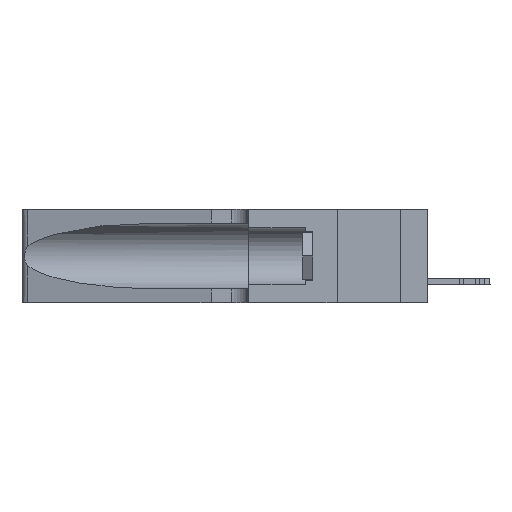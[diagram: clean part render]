
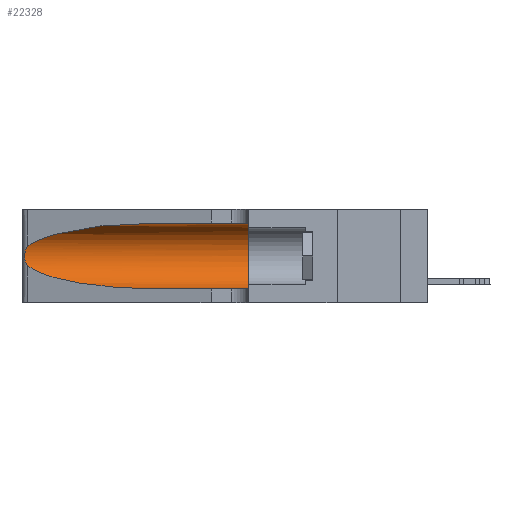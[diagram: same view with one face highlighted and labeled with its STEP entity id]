
A CAD part, left-side view. The second image highlights one B-rep face of the part: STEP entity #22328.
In plain terms, the highlighted cylindrical face has radius 3.308 mm (diameter 6.617 mm), a partial arc.
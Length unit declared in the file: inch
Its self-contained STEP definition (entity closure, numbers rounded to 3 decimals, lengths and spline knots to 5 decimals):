
#170 = CARTESIAN_POINT ( 'NONE',  ( 0.1305, 0.72297, 0.05475 ) ) ;
#657 = LINE ( 'NONE', #12753, #15418 ) ;
#1039 = CARTESIAN_POINT ( 'NONE',  ( 0.25487, 1.22718, 0.14631 ) ) ;
#1670 = VERTEX_POINT ( 'NONE', #14358 ) ;
#2131 = AXIS2_PLACEMENT_3D ( 'NONE', #8786, #8942, #35774 ) ;
#4303 = EDGE_CURVE ( 'NONE', #12746, #25970, #12121, .T. ) ;
#4893 = CARTESIAN_POINT ( 'NONE',  ( 0.26018, 1.23835, 0.19895 ) ) ;
#6240 = FACE_OUTER_BOUND ( 'NONE', #11976, .T. ) ;
#8786 = CARTESIAN_POINT ( 'NONE',  ( 0.1305, 0.35, 0.185 ) ) ;
#8942 = DIRECTION ( 'NONE',  ( 0., 1., 0. ) ) ;
#9228 = DIRECTION ( 'NONE',  ( 0., -1., 0. ) ) ;
#10283 = ORIENTED_EDGE ( 'NONE', *, *, #4303, .F. ) ;
#11208 = DIRECTION ( 'NONE',  ( 0., -1., 0. ) ) ;
#11501 = CARTESIAN_POINT ( 'NONE',  ( 0.26017, 1.23833, 0.17102 ) ) ;
#11976 = EDGE_LOOP ( 'NONE', ( #29747, #21127, #13258, #29971, #10283, #15335 ) ) ;
#12121 = CIRCLE ( 'NONE', #2131, 0.13025 ) ;
#12572 = VERTEX_POINT ( 'NONE', #23150 ) ;
#12648 = VERTEX_POINT ( 'NONE', #15117 ) ;
#12746 = VERTEX_POINT ( 'NONE', #41838 ) ;
#12753 = CARTESIAN_POINT ( 'NONE',  ( 0.1305, 1.61858, 0.05475 ) ) ;
#13258 = ORIENTED_EDGE ( 'NONE', *, *, #41507, .T. ) ;
#13763 = CARTESIAN_POINT ( 'NONE',  ( 0.1305, 0.72297, 0.31525 ) ) ;
#14358 = CARTESIAN_POINT ( 'NONE',  ( 0.25487, 1.22718, 0.14631 ) ) ;
#14885 = CARTESIAN_POINT ( 'NONE',  ( 0.25789, 1.23486, 0.15765 ) ) ;
#15117 = CARTESIAN_POINT ( 'NONE',  ( 0.25487, 1.22718, 0.22369 ) ) ;
#15335 = ORIENTED_EDGE ( 'NONE', *, *, #25459, .F. ) ;
#15418 = VECTOR ( 'NONE', #9228, 39.37008 ) ;
#16568 = LINE ( 'NONE', #31150, #32900 ) ;
#16634 = CARTESIAN_POINT ( 'NONE',  ( 0.18966, 0.96281, 0.31525 ) ) ;
#17762 = B_SPLINE_CURVE_WITH_KNOTS ( 'NONE', 3,
 ( #21868, #42118, #39004, #28950, #18759, #4893, #42271, #35710, #11501, #32197, #14885, #18617, #18314, #42435 ),
 .UNSPECIFIED., .F., .F.,
 ( 4, 2, 2, 2, 2, 2, 4 ),
 ( 0., 0.00027, 0.00053, 0.00107, 0.0016, 0.00187, 0.00214 ),
 .UNSPECIFIED. ) ;
#17767 = CYLINDRICAL_SURFACE ( 'NONE', #22384, 0.13025 ) ;
#18314 = CARTESIAN_POINT ( 'NONE',  ( 0.25555, 1.22993, 0.14849 ) ) ;
#18617 = CARTESIAN_POINT ( 'NONE',  ( 0.25639, 1.23186, 0.15144 ) ) ;
#18759 = CARTESIAN_POINT ( 'NONE',  ( 0.25854, 1.2359, 0.20912 ) ) ;
#19297 = CARTESIAN_POINT ( 'NONE',  ( 0.1305, 0.35, 0.05475 ) ) ;
#19692 = EDGE_CURVE ( 'NONE', #12572, #25970, #657, .T. ) ;
#20511 =( BOUNDED_CURVE ( )  B_SPLINE_CURVE ( 3, ( #1039, #24643, #34062, #170 ),
 .UNSPECIFIED., .F., .F. ) 
 B_SPLINE_CURVE_WITH_KNOTS ( ( 4, 4 ),
 ( 3.44316, 4.71239 ),
 .UNSPECIFIED. ) 
 CURVE ( )  GEOMETRIC_REPRESENTATION_ITEM ( )  RATIONAL_B_SPLINE_CURVE ( ( 1., 0.87, 0.87, 1. ) ) 
 REPRESENTATION_ITEM ( '' )  );
#21127 = ORIENTED_EDGE ( 'NONE', *, *, #36925, .T. ) ;
#21868 = CARTESIAN_POINT ( 'NONE',  ( 0.25487, 1.22718, 0.22369 ) ) ;
#22328 = ADVANCED_FACE ( 'NONE', ( #6240 ), #17767, .F. ) ;
#22384 = AXIS2_PLACEMENT_3D ( 'NONE', #37200, #41311, #41622 ) ;
#23150 = CARTESIAN_POINT ( 'NONE',  ( 0.1305, 0.72297, 0.05475 ) ) ;
#24643 = CARTESIAN_POINT ( 'NONE',  ( 0.2373, 1.15595, 0.08982 ) ) ;
#25459 = EDGE_CURVE ( 'NONE', #35437, #12746, #16568, .T. ) ;
#25970 = VERTEX_POINT ( 'NONE', #19297 ) ;
#28950 = CARTESIAN_POINT ( 'NONE',  ( 0.25787, 1.23484, 0.2124 ) ) ;
#29747 = ORIENTED_EDGE ( 'NONE', *, *, #37777, .T. ) ;
#29971 = ORIENTED_EDGE ( 'NONE', *, *, #19692, .T. ) ;
#30467 = CARTESIAN_POINT ( 'NONE',  ( 0.25487, 1.22718, 0.22369 ) ) ;
#31150 = CARTESIAN_POINT ( 'NONE',  ( 0.1305, 1.61858, 0.31525 ) ) ;
#32197 = CARTESIAN_POINT ( 'NONE',  ( 0.25856, 1.23593, 0.16098 ) ) ;
#32900 = VECTOR ( 'NONE', #11208, 39.37008 ) ;
#33621 = CARTESIAN_POINT ( 'NONE',  ( 0.2373, 1.15595, 0.28018 ) ) ;
#34062 = CARTESIAN_POINT ( 'NONE',  ( 0.18966, 0.96281, 0.05475 ) ) ;
#34280 =( BOUNDED_CURVE ( )  B_SPLINE_CURVE ( 3, ( #39825, #16634, #33621, #30467 ),
 .UNSPECIFIED., .F., .F. ) 
 B_SPLINE_CURVE_WITH_KNOTS ( ( 4, 4 ),
 ( 1.5708, 2.84003 ),
 .UNSPECIFIED. ) 
 CURVE ( )  GEOMETRIC_REPRESENTATION_ITEM ( )  RATIONAL_B_SPLINE_CURVE ( ( 1., 0.87, 0.87, 1. ) ) 
 REPRESENTATION_ITEM ( '' )  );
#35437 = VERTEX_POINT ( 'NONE', #13763 ) ;
#35710 = CARTESIAN_POINT ( 'NONE',  ( 0.26075, 1.23896, 0.178 ) ) ;
#35774 = DIRECTION ( 'NONE',  ( 0., 0., 1. ) ) ;
#36925 = EDGE_CURVE ( 'NONE', #12648, #1670, #17762, .T. ) ;
#37200 = CARTESIAN_POINT ( 'NONE',  ( 0.1305, 1.61858, 0.185 ) ) ;
#37777 = EDGE_CURVE ( 'NONE', #35437, #12648, #34280, .T. ) ;
#39004 = CARTESIAN_POINT ( 'NONE',  ( 0.25639, 1.23184, 0.21858 ) ) ;
#39825 = CARTESIAN_POINT ( 'NONE',  ( 0.1305, 0.72297, 0.31525 ) ) ;
#41311 = DIRECTION ( 'NONE',  ( 0., -1., 0. ) ) ;
#41507 = EDGE_CURVE ( 'NONE', #1670, #12572, #20511, .T. ) ;
#41622 = DIRECTION ( 'NONE',  ( 0., 0., -1. ) ) ;
#41838 = CARTESIAN_POINT ( 'NONE',  ( 0.1305, 0.35, 0.31525 ) ) ;
#42118 = CARTESIAN_POINT ( 'NONE',  ( 0.25555, 1.22994, 0.2215 ) ) ;
#42271 = CARTESIAN_POINT ( 'NONE',  ( 0.26075, 1.23896, 0.19203 ) ) ;
#42435 = CARTESIAN_POINT ( 'NONE',  ( 0.25487, 1.22718, 0.14631 ) ) ;
